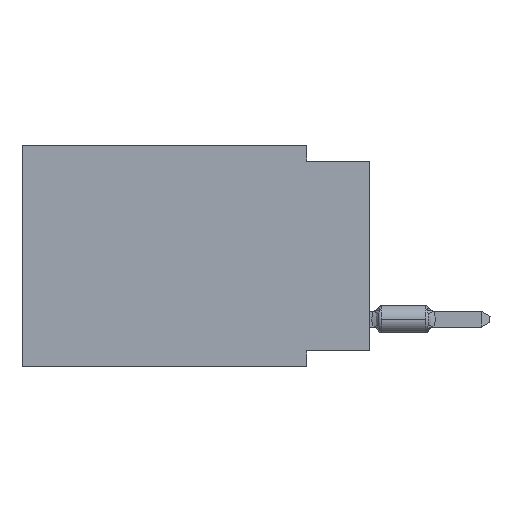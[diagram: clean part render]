
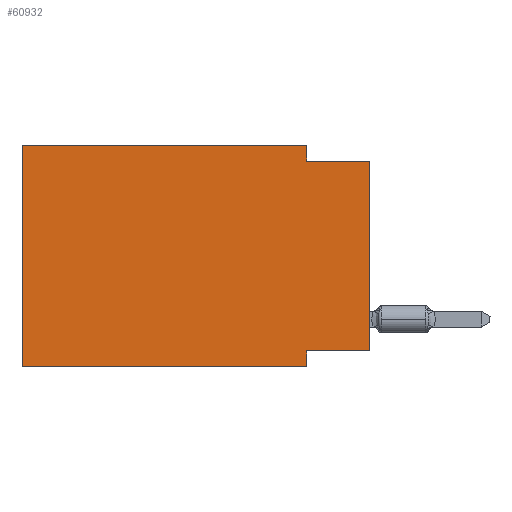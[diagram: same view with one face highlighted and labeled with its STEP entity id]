
A CAD part, left-side view. The second image highlights one B-rep face of the part: STEP entity #60932.
In plain terms, the highlighted planar face has unit normal (-1, 0, 0).
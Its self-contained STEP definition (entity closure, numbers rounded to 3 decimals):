
#3529 = EDGE_CURVE ( 'NONE', #75914, #15730, #85587, .T. ) ;
#5256 = CARTESIAN_POINT ( 'NONE',  ( 0., 2.54, -0.635 ) ) ;
#6553 = DIRECTION ( 'NONE',  ( 0., 0., -1. ) ) ;
#7210 = CARTESIAN_POINT ( 'NONE',  ( 0., 13.97, 0. ) ) ;
#9730 = EDGE_CURVE ( 'NONE', #86575, #82125, #68194, .T. ) ;
#10219 = CARTESIAN_POINT ( 'NONE',  ( 0., 2.54, 0. ) ) ;
#12300 = ORIENTED_EDGE ( 'NONE', *, *, #17372, .T. ) ;
#15165 = VERTEX_POINT ( 'NONE', #62532 ) ;
#15428 = PLANE ( 'NONE',  #75791 ) ;
#15730 = VERTEX_POINT ( 'NONE', #10219 ) ;
#16860 = CARTESIAN_POINT ( 'NONE',  ( 0., 13.97, 0. ) ) ;
#17372 = EDGE_CURVE ( 'NONE', #15165, #25816, #34096, .T. ) ;
#17457 = CARTESIAN_POINT ( 'NONE',  ( 0., 0., 0. ) ) ;
#17872 = VECTOR ( 'NONE', #32866, 1000. ) ;
#22474 = VERTEX_POINT ( 'NONE', #73603 ) ;
#23560 = CARTESIAN_POINT ( 'NONE',  ( 0., 0., -0.635 ) ) ;
#25816 = VERTEX_POINT ( 'NONE', #23560 ) ;
#26158 = EDGE_CURVE ( 'NONE', #86575, #75914, #36454, .T. ) ;
#26193 = ORIENTED_EDGE ( 'NONE', *, *, #54910, .F. ) ;
#27984 = LINE ( 'NONE', #57308, #84193 ) ;
#28178 = VERTEX_POINT ( 'NONE', #5256 ) ;
#30734 = VECTOR ( 'NONE', #68681, 1000. ) ;
#32866 = DIRECTION ( 'NONE',  ( 0., 0., -1. ) ) ;
#34096 = LINE ( 'NONE', #17457, #60559 ) ;
#35557 = DIRECTION ( 'NONE',  ( 0., -1., 0. ) ) ;
#36454 = LINE ( 'NONE', #88359, #87370 ) ;
#37689 = ORIENTED_EDGE ( 'NONE', *, *, #78841, .F. ) ;
#41957 = ORIENTED_EDGE ( 'NONE', *, *, #80812, .F. ) ;
#43043 = CARTESIAN_POINT ( 'NONE',  ( 0., 13.97, 0. ) ) ;
#44024 = CARTESIAN_POINT ( 'NONE',  ( 0., 13.97, -8.89 ) ) ;
#45856 = LINE ( 'NONE', #76624, #17872 ) ;
#46803 = CARTESIAN_POINT ( 'NONE',  ( 0., 0., -0.635 ) ) ;
#48468 = VECTOR ( 'NONE', #6553, 1000. ) ;
#51513 = DIRECTION ( 'NONE',  ( 0., 1., 0. ) ) ;
#54910 = EDGE_CURVE ( 'NONE', #15165, #22474, #27984, .T. ) ;
#55101 = VECTOR ( 'NONE', #74708, 1000. ) ;
#56869 = CARTESIAN_POINT ( 'NONE',  ( 0., 2.54, -8.89 ) ) ;
#57308 = CARTESIAN_POINT ( 'NONE',  ( 0., 0., -8.255 ) ) ;
#60514 = CARTESIAN_POINT ( 'NONE',  ( 0., 13.97, -8.89 ) ) ;
#60559 = VECTOR ( 'NONE', #83798, 1000. ) ;
#60622 = VECTOR ( 'NONE', #35557, 1000. ) ;
#60932 = ADVANCED_FACE ( 'NONE', ( #82237 ), #15428, .F. ) ;
#62532 = CARTESIAN_POINT ( 'NONE',  ( 0., 0., -8.255 ) ) ;
#63153 = EDGE_CURVE ( 'NONE', #22474, #82125, #72395, .T. ) ;
#68194 = LINE ( 'NONE', #60514, #30734 ) ;
#68681 = DIRECTION ( 'NONE',  ( 0., -1., 0. ) ) ;
#68916 = ORIENTED_EDGE ( 'NONE', *, *, #3529, .F. ) ;
#72395 = LINE ( 'NONE', #73356, #48468 ) ;
#73356 = CARTESIAN_POINT ( 'NONE',  ( 0., 2.54, -8.89 ) ) ;
#73460 = EDGE_LOOP ( 'NONE', ( #12300, #37689, #41957, #68916, #83600, #78202, #91911, #26193 ) ) ;
#73603 = CARTESIAN_POINT ( 'NONE',  ( 0., 2.54, -8.255 ) ) ;
#74708 = DIRECTION ( 'NONE',  ( 0., -1., 0. ) ) ;
#75791 = AXIS2_PLACEMENT_3D ( 'NONE', #16860, #88510, #81758 ) ;
#75914 = VERTEX_POINT ( 'NONE', #43043 ) ;
#76624 = CARTESIAN_POINT ( 'NONE',  ( 0., 2.54, 0. ) ) ;
#78202 = ORIENTED_EDGE ( 'NONE', *, *, #9730, .T. ) ;
#78841 = EDGE_CURVE ( 'NONE', #28178, #25816, #88668, .T. ) ;
#80812 = EDGE_CURVE ( 'NONE', #15730, #28178, #45856, .T. ) ;
#81758 = DIRECTION ( 'NONE',  ( 0., 0., -1. ) ) ;
#82125 = VERTEX_POINT ( 'NONE', #56869 ) ;
#82237 = FACE_OUTER_BOUND ( 'NONE', #73460, .T. ) ;
#83600 = ORIENTED_EDGE ( 'NONE', *, *, #26158, .F. ) ;
#83798 = DIRECTION ( 'NONE',  ( 0., 0., 1. ) ) ;
#84193 = VECTOR ( 'NONE', #51513, 1000. ) ;
#85587 = LINE ( 'NONE', #7210, #60622 ) ;
#86575 = VERTEX_POINT ( 'NONE', #44024 ) ;
#87370 = VECTOR ( 'NONE', #95107, 1000. ) ;
#88359 = CARTESIAN_POINT ( 'NONE',  ( 0., 13.97, 0. ) ) ;
#88510 = DIRECTION ( 'NONE',  ( 1., 0., 0. ) ) ;
#88668 = LINE ( 'NONE', #46803, #55101 ) ;
#91911 = ORIENTED_EDGE ( 'NONE', *, *, #63153, .F. ) ;
#95107 = DIRECTION ( 'NONE',  ( 0., 0., 1. ) ) ;
